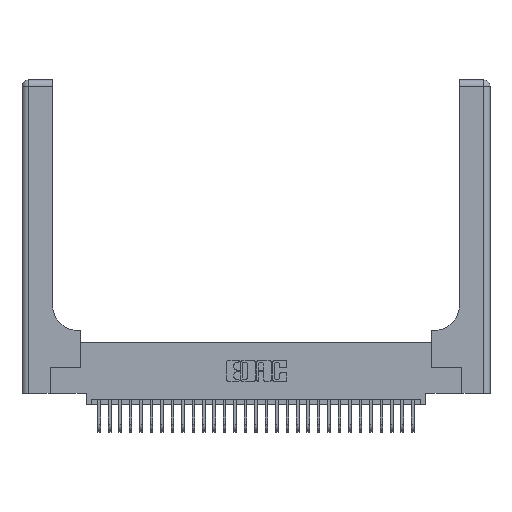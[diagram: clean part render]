
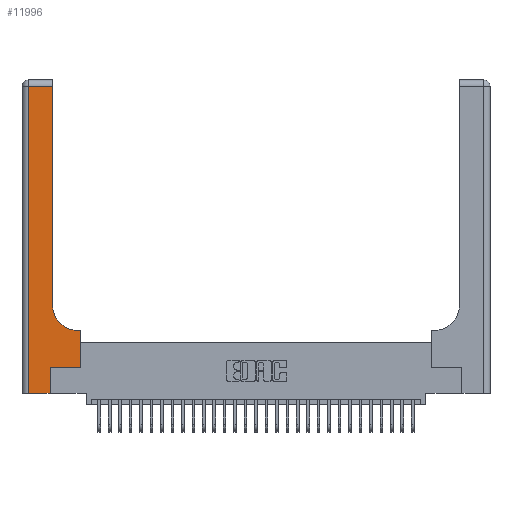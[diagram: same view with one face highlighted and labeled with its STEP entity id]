
A CAD part, top view. The second image highlights one B-rep face of the part: STEP entity #11996.
In plain terms, the highlighted planar face has unit normal (0, 0, 1).
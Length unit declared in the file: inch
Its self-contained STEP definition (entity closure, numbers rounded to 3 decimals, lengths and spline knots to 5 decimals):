
#73 = VERTEX_POINT ( 'NONE', #3664 ) ;
#505 = LINE ( 'NONE', #22753, #9208 ) ;
#1002 = VERTEX_POINT ( 'NONE', #22939 ) ;
#1509 = VERTEX_POINT ( 'NONE', #9243 ) ;
#1733 = VECTOR ( 'NONE', #14176, 39.37008 ) ;
#2607 = ORIENTED_EDGE ( 'NONE', *, *, #23262, .T. ) ;
#3559 = DIRECTION ( 'NONE',  ( -1., 0., 0. ) ) ;
#3664 = CARTESIAN_POINT ( 'NONE',  ( 0.06, 2.94, 0.37 ) ) ;
#3678 = LINE ( 'NONE', #31441, #29832 ) ;
#4015 = ORIENTED_EDGE ( 'NONE', *, *, #11391, .T. ) ;
#4304 = VERTEX_POINT ( 'NONE', #6334 ) ;
#5160 = VECTOR ( 'NONE', #11876, 39.37008 ) ;
#6052 = FACE_OUTER_BOUND ( 'NONE', #28062, .T. ) ;
#6161 = VERTEX_POINT ( 'NONE', #11713 ) ;
#6334 = CARTESIAN_POINT ( 'NONE',  ( 0.2915, 2.94, 0.37 ) ) ;
#6431 = EDGE_CURVE ( 'NONE', #22466, #4304, #15219, .T. ) ;
#6663 = PLANE ( 'NONE',  #22339 ) ;
#6734 = EDGE_CURVE ( 'NONE', #32097, #1002, #29029, .T. ) ;
#7055 = VECTOR ( 'NONE', #23089, 39.37008 ) ;
#7471 = CARTESIAN_POINT ( 'NONE',  ( 0.2915, 0.85, 0.37 ) ) ;
#7690 = VECTOR ( 'NONE', #3559, 39.37008 ) ;
#8237 = ORIENTED_EDGE ( 'NONE', *, *, #25920, .T. ) ;
#8848 = VECTOR ( 'NONE', #32461, 39.37008 ) ;
#9208 = VECTOR ( 'NONE', #12406, 39.37008 ) ;
#9243 = CARTESIAN_POINT ( 'NONE',  ( 0.5415, 0.6, 0.37 ) ) ;
#9381 = CARTESIAN_POINT ( 'NONE',  ( 0.5585, 0.25, 0.37 ) ) ;
#9912 = VERTEX_POINT ( 'NONE', #25067 ) ;
#10083 = DIRECTION ( 'NONE',  ( 0., 0., -1. ) ) ;
#11269 = ORIENTED_EDGE ( 'NONE', *, *, #6734, .T. ) ;
#11391 = EDGE_CURVE ( 'NONE', #9912, #1509, #20695, .T. ) ;
#11713 = CARTESIAN_POINT ( 'NONE',  ( 0.269, 0.25, 0.37 ) ) ;
#11876 = DIRECTION ( 'NONE',  ( 0., 1., 0. ) ) ;
#11996 = ADVANCED_FACE ( 'NONE', ( #6052 ), #6663, .F. ) ;
#12071 = EDGE_CURVE ( 'NONE', #6161, #22087, #505, .T. ) ;
#12406 = DIRECTION ( 'NONE',  ( 1., 0., 0. ) ) ;
#12439 = CIRCLE ( 'NONE', #27483, 0.25 ) ;
#12831 = ORIENTED_EDGE ( 'NONE', *, *, #28802, .T. ) ;
#14102 = EDGE_CURVE ( 'NONE', #4304, #73, #32061, .T. ) ;
#14176 = DIRECTION ( 'NONE',  ( 0., 1., 0. ) ) ;
#14188 = DIRECTION ( 'NONE',  ( 0., 0., -1. ) ) ;
#15004 = ORIENTED_EDGE ( 'NONE', *, *, #14102, .T. ) ;
#15219 = LINE ( 'NONE', #25751, #1733 ) ;
#16025 = DIRECTION ( 'NONE',  ( 0., -1., 0. ) ) ;
#16039 = VECTOR ( 'NONE', #29394, 39.37008 ) ;
#16450 = EDGE_CURVE ( 'NONE', #22087, #9912, #22730, .T. ) ;
#16924 = DIRECTION ( 'NONE',  ( -1., 0., 0. ) ) ;
#17466 = ORIENTED_EDGE ( 'NONE', *, *, #6431, .T. ) ;
#17820 = CARTESIAN_POINT ( 'NONE',  ( 0., 2.94, 0.37 ) ) ;
#17985 = CARTESIAN_POINT ( 'NONE',  ( 0.5585, 0.25, 0.37 ) ) ;
#19764 = CARTESIAN_POINT ( 'NONE',  ( 0.5415, 0.85, 0.37 ) ) ;
#19980 = ORIENTED_EDGE ( 'NONE', *, *, #12071, .T. ) ;
#20695 = LINE ( 'NONE', #29227, #7690 ) ;
#22087 = VERTEX_POINT ( 'NONE', #17985 ) ;
#22327 = CARTESIAN_POINT ( 'NONE',  ( 0.269, 0., 0.37 ) ) ;
#22339 = AXIS2_PLACEMENT_3D ( 'NONE', #24628, #14188, #16924 ) ;
#22409 = DIRECTION ( 'NONE',  ( 1., 0., 0. ) ) ;
#22466 = VERTEX_POINT ( 'NONE', #7471 ) ;
#22730 = LINE ( 'NONE', #9381, #16039 ) ;
#22753 = CARTESIAN_POINT ( 'NONE',  ( 0.269, 0.25, 0.37 ) ) ;
#22939 = CARTESIAN_POINT ( 'NONE',  ( 0.269, 0., 0.37 ) ) ;
#23089 = DIRECTION ( 'NONE',  ( -1., 0., 0. ) ) ;
#23262 = EDGE_CURVE ( 'NONE', #73, #32097, #3678, .T. ) ;
#24628 = CARTESIAN_POINT ( 'NONE',  ( 0., 3., 0.37 ) ) ;
#25067 = CARTESIAN_POINT ( 'NONE',  ( 0.5585, 0.6, 0.37 ) ) ;
#25694 = LINE ( 'NONE', #22327, #5160 ) ;
#25751 = CARTESIAN_POINT ( 'NONE',  ( 0.2915, 3., 0.37 ) ) ;
#25920 = EDGE_CURVE ( 'NONE', #1509, #22466, #12439, .T. ) ;
#27317 = CARTESIAN_POINT ( 'NONE',  ( 0., 0., 0.37 ) ) ;
#27483 = AXIS2_PLACEMENT_3D ( 'NONE', #19764, #10083, #22409 ) ;
#28062 = EDGE_LOOP ( 'NONE', ( #17466, #15004, #2607, #11269, #12831, #19980, #32067, #4015, #8237 ) ) ;
#28802 = EDGE_CURVE ( 'NONE', #1002, #6161, #25694, .T. ) ;
#29029 = LINE ( 'NONE', #27317, #8848 ) ;
#29227 = CARTESIAN_POINT ( 'NONE',  ( 0.2915, 0.6, 0.37 ) ) ;
#29394 = DIRECTION ( 'NONE',  ( 0., 1., 0. ) ) ;
#29832 = VECTOR ( 'NONE', #16025, 39.37008 ) ;
#29868 = CARTESIAN_POINT ( 'NONE',  ( 0.06, 0., 0.37 ) ) ;
#31441 = CARTESIAN_POINT ( 'NONE',  ( 0.06, 3., 0.37 ) ) ;
#32061 = LINE ( 'NONE', #17820, #7055 ) ;
#32067 = ORIENTED_EDGE ( 'NONE', *, *, #16450, .T. ) ;
#32097 = VERTEX_POINT ( 'NONE', #29868 ) ;
#32461 = DIRECTION ( 'NONE',  ( 1., 0., 0. ) ) ;
